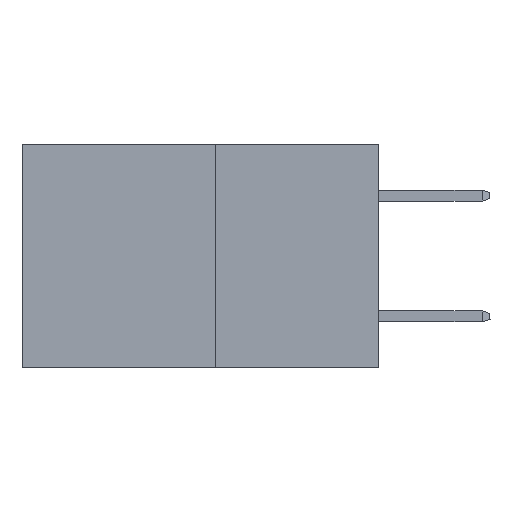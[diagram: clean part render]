
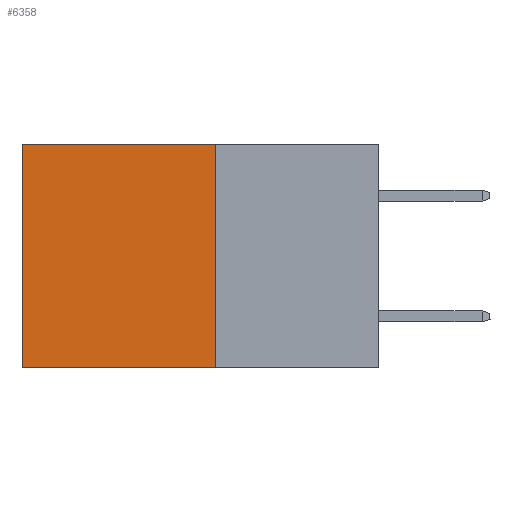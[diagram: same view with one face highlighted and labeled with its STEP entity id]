
A CAD part, left-side view. The second image highlights one B-rep face of the part: STEP entity #6358.
In plain terms, the highlighted planar face has unit normal (-1, 0, 0).
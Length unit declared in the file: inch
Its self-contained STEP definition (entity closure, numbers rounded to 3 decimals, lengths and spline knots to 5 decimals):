
#46 = PLANE ( 'NONE',  #8860 ) ;
#481 = CARTESIAN_POINT ( 'NONE',  ( 0.277, 0.59, 0. ) ) ;
#815 = EDGE_LOOP ( 'NONE', ( #10196, #7934, #5997, #11670 ) ) ;
#1184 = LINE ( 'NONE', #18602, #19635 ) ;
#3290 = VERTEX_POINT ( 'NONE', #481 ) ;
#5016 = CARTESIAN_POINT ( 'NONE',  ( 0.277, 0.27, -0.37 ) ) ;
#5694 = LINE ( 'NONE', #5016, #14123 ) ;
#5817 = EDGE_CURVE ( 'NONE', #5832, #12316, #7902, .T. ) ;
#5832 = VERTEX_POINT ( 'NONE', #12035 ) ;
#5997 = ORIENTED_EDGE ( 'NONE', *, *, #17777, .F. ) ;
#6174 = FACE_OUTER_BOUND ( 'NONE', #815, .T. ) ;
#6358 = ADVANCED_FACE ( 'NONE', ( #6174 ), #46, .F. ) ;
#7333 = VECTOR ( 'NONE', #12272, 39.37008 ) ;
#7902 = LINE ( 'NONE', #13009, #7333 ) ;
#7934 = ORIENTED_EDGE ( 'NONE', *, *, #5817, .F. ) ;
#8860 = AXIS2_PLACEMENT_3D ( 'NONE', #22824, #22371, #22327 ) ;
#9257 = CARTESIAN_POINT ( 'NONE',  ( 0.277, 0.59, -0.37 ) ) ;
#10196 = ORIENTED_EDGE ( 'NONE', *, *, #17533, .T. ) ;
#10743 = CARTESIAN_POINT ( 'NONE',  ( 0.277, 0.27, 0. ) ) ;
#11211 = DIRECTION ( 'NONE',  ( 0., 1., 0. ) ) ;
#11501 = VERTEX_POINT ( 'NONE', #10743 ) ;
#11670 = ORIENTED_EDGE ( 'NONE', *, *, #13663, .T. ) ;
#12035 = CARTESIAN_POINT ( 'NONE',  ( 0.277, 0.27, -0.37 ) ) ;
#12272 = DIRECTION ( 'NONE',  ( 0., 1., 0. ) ) ;
#12316 = VERTEX_POINT ( 'NONE', #9257 ) ;
#13009 = CARTESIAN_POINT ( 'NONE',  ( 0.277, 0.27, -0.37 ) ) ;
#13205 = LINE ( 'NONE', #20044, #16790 ) ;
#13663 = EDGE_CURVE ( 'NONE', #11501, #3290, #13205, .T. ) ;
#14123 = VECTOR ( 'NONE', #15744, 39.37008 ) ;
#15744 = DIRECTION ( 'NONE',  ( 0., 0., -1. ) ) ;
#16790 = VECTOR ( 'NONE', #11211, 39.37008 ) ;
#17533 = EDGE_CURVE ( 'NONE', #3290, #12316, #1184, .T. ) ;
#17777 = EDGE_CURVE ( 'NONE', #11501, #5832, #5694, .T. ) ;
#18602 = CARTESIAN_POINT ( 'NONE',  ( 0.277, 0.59, -0.37 ) ) ;
#19635 = VECTOR ( 'NONE', #20378, 39.37008 ) ;
#20044 = CARTESIAN_POINT ( 'NONE',  ( 0.277, 0.27, 0. ) ) ;
#20378 = DIRECTION ( 'NONE',  ( 0., 0., -1. ) ) ;
#22327 = DIRECTION ( 'NONE',  ( 0., 0., -1. ) ) ;
#22371 = DIRECTION ( 'NONE',  ( 1., 0., 0. ) ) ;
#22824 = CARTESIAN_POINT ( 'NONE',  ( 0.277, 0.27, -0.37 ) ) ;
